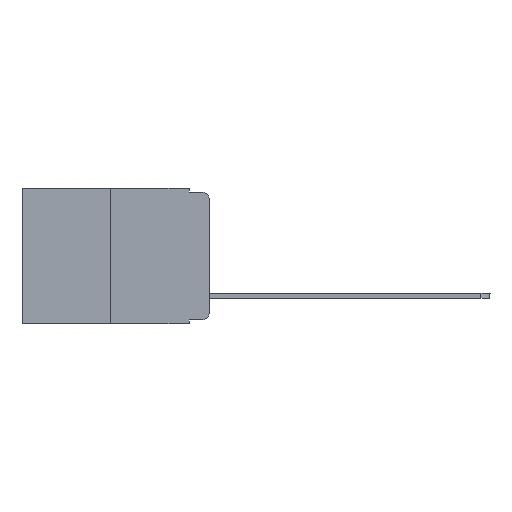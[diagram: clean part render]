
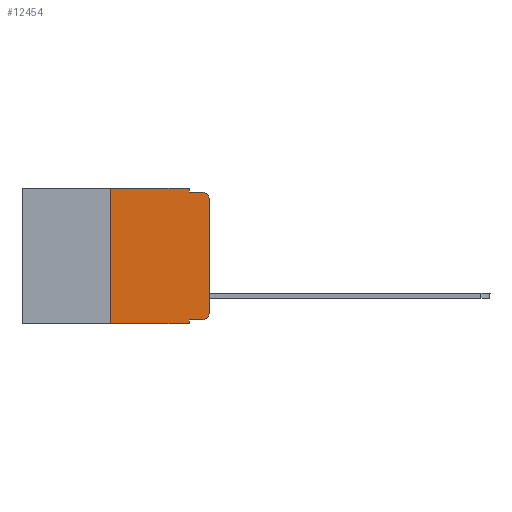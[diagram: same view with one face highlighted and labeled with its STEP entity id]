
A CAD part, left-side view. The second image highlights one B-rep face of the part: STEP entity #12454.
In plain terms, the highlighted planar face has unit normal (-1, 0, 0).
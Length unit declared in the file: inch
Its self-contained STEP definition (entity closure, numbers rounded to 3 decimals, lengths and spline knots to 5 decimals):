
#267 = DIRECTION ( 'NONE',  ( 0., 0., -1. ) ) ;
#279 = FACE_OUTER_BOUND ( 'NONE', #4727, .T. ) ;
#537 = CARTESIAN_POINT ( 'NONE',  ( 0., 0.25, -0.343 ) ) ;
#823 = CARTESIAN_POINT ( 'NONE',  ( 0., 0.051, -0.01 ) ) ;
#937 = DIRECTION ( 'NONE',  ( 0., 0., -1. ) ) ;
#1049 = VECTOR ( 'NONE', #5866, 39.37008 ) ;
#1143 = LINE ( 'NONE', #20910, #19059 ) ;
#1323 = CARTESIAN_POINT ( 'NONE',  ( 0., 0.02, -0.333 ) ) ;
#1586 = ORIENTED_EDGE ( 'NONE', *, *, #7653, .T. ) ;
#2081 = VECTOR ( 'NONE', #16300, 39.37008 ) ;
#2271 = VERTEX_POINT ( 'NONE', #14777 ) ;
#2594 = EDGE_CURVE ( 'NONE', #22328, #10674, #8433, .T. ) ;
#2928 = PLANE ( 'NONE',  #20676 ) ;
#3011 = ORIENTED_EDGE ( 'NONE', *, *, #5702, .F. ) ;
#3160 = CARTESIAN_POINT ( 'NONE',  ( 0., 0., -0.313 ) ) ;
#3504 = EDGE_CURVE ( 'NONE', #10674, #11081, #6456, .T. ) ;
#3681 = DIRECTION ( 'NONE',  ( 0., 0., 1. ) ) ;
#3703 = ORIENTED_EDGE ( 'NONE', *, *, #4003, .F. ) ;
#3707 = EDGE_CURVE ( 'NONE', #8297, #18809, #19769, .T. ) ;
#3853 = DIRECTION ( 'NONE',  ( -1., 0., 0. ) ) ;
#4003 = EDGE_CURVE ( 'NONE', #18809, #17124, #11344, .T. ) ;
#4216 = CARTESIAN_POINT ( 'NONE',  ( 0., 0.051, 0. ) ) ;
#4232 = DIRECTION ( 'NONE',  ( 0., 0., -1. ) ) ;
#4534 = DIRECTION ( 'NONE',  ( -1., 0., 0. ) ) ;
#4727 = EDGE_LOOP ( 'NONE', ( #17742, #10863, #9077, #3703, #17565, #3011, #20948, #12377, #1586, #6518 ) ) ;
#4800 = EDGE_CURVE ( 'NONE', #17124, #2271, #5360, .T. ) ;
#5360 = LINE ( 'NONE', #823, #9434 ) ;
#5702 = EDGE_CURVE ( 'NONE', #21462, #8297, #20244, .T. ) ;
#5766 = EDGE_CURVE ( 'NONE', #17418, #16023, #17217, .T. ) ;
#5866 = DIRECTION ( 'NONE',  ( 0., -1., 0. ) ) ;
#5897 = CARTESIAN_POINT ( 'NONE',  ( 0., 0.25, 0. ) ) ;
#6114 = CARTESIAN_POINT ( 'NONE',  ( 0., 0.02, -0.313 ) ) ;
#6185 = VECTOR ( 'NONE', #3681, 39.37008 ) ;
#6456 = LINE ( 'NONE', #17328, #6185 ) ;
#6518 = ORIENTED_EDGE ( 'NONE', *, *, #2594, .T. ) ;
#7080 = EDGE_CURVE ( 'NONE', #11081, #2271, #10148, .T. ) ;
#7615 = AXIS2_PLACEMENT_3D ( 'NONE', #17784, #3853, #267 ) ;
#7647 = CARTESIAN_POINT ( 'NONE',  ( 0., 0.051, -0.01 ) ) ;
#7653 = EDGE_CURVE ( 'NONE', #17418, #22328, #1143, .T. ) ;
#7744 = DIRECTION ( 'NONE',  ( 0., -1., 0. ) ) ;
#8297 = VERTEX_POINT ( 'NONE', #21191 ) ;
#8433 = CIRCLE ( 'NONE', #11158, 0.02 ) ;
#9013 = CARTESIAN_POINT ( 'NONE',  ( 0., 0.051, -0.343 ) ) ;
#9015 = CARTESIAN_POINT ( 'NONE',  ( 0., 0.051, -0.333 ) ) ;
#9077 = ORIENTED_EDGE ( 'NONE', *, *, #4800, .F. ) ;
#9255 = DIRECTION ( 'NONE',  ( 0., 0., 1. ) ) ;
#9434 = VECTOR ( 'NONE', #7744, 39.37008 ) ;
#9461 = EDGE_CURVE ( 'NONE', #21462, #16023, #21639, .T. ) ;
#9696 = CARTESIAN_POINT ( 'NONE',  ( 0., 0.473, 0. ) ) ;
#10148 = CIRCLE ( 'NONE', #7615, 0.02 ) ;
#10589 = DIRECTION ( 'NONE',  ( 0., -1., 0. ) ) ;
#10674 = VERTEX_POINT ( 'NONE', #3160 ) ;
#10863 = ORIENTED_EDGE ( 'NONE', *, *, #7080, .T. ) ;
#11081 = VERTEX_POINT ( 'NONE', #14730 ) ;
#11119 = CARTESIAN_POINT ( 'NONE',  ( 0., 0.051, 0. ) ) ;
#11125 = CARTESIAN_POINT ( 'NONE',  ( 0., 0.051, 0. ) ) ;
#11158 = AXIS2_PLACEMENT_3D ( 'NONE', #6114, #4534, #16641 ) ;
#11344 = LINE ( 'NONE', #4216, #17839 ) ;
#12365 = VECTOR ( 'NONE', #4232, 39.37008 ) ;
#12377 = ORIENTED_EDGE ( 'NONE', *, *, #5766, .F. ) ;
#12454 = ADVANCED_FACE ( 'NONE', ( #279 ), #2928, .F. ) ;
#12939 = DIRECTION ( 'NONE',  ( 0., 0., -1. ) ) ;
#14519 = VECTOR ( 'NONE', #9255, 39.37008 ) ;
#14730 = CARTESIAN_POINT ( 'NONE',  ( 0., 0., -0.03 ) ) ;
#14777 = CARTESIAN_POINT ( 'NONE',  ( 0., 0.02, -0.01 ) ) ;
#15057 = DIRECTION ( 'NONE',  ( 1., 0., 0. ) ) ;
#16023 = VERTEX_POINT ( 'NONE', #9013 ) ;
#16244 = CARTESIAN_POINT ( 'NONE',  ( 0., 0.473, 0. ) ) ;
#16300 = DIRECTION ( 'NONE',  ( 0., -1., 0. ) ) ;
#16641 = DIRECTION ( 'NONE',  ( 0., 0., -1. ) ) ;
#17124 = VERTEX_POINT ( 'NONE', #7647 ) ;
#17217 = LINE ( 'NONE', #11119, #12365 ) ;
#17328 = CARTESIAN_POINT ( 'NONE',  ( 0., 0., 0. ) ) ;
#17418 = VERTEX_POINT ( 'NONE', #9015 ) ;
#17565 = ORIENTED_EDGE ( 'NONE', *, *, #3707, .F. ) ;
#17742 = ORIENTED_EDGE ( 'NONE', *, *, #3504, .T. ) ;
#17784 = CARTESIAN_POINT ( 'NONE',  ( 0., 0.02, -0.03 ) ) ;
#17839 = VECTOR ( 'NONE', #12939, 39.37008 ) ;
#17892 = CARTESIAN_POINT ( 'NONE',  ( 0., 0.473, -0.343 ) ) ;
#18809 = VERTEX_POINT ( 'NONE', #11125 ) ;
#19059 = VECTOR ( 'NONE', #10589, 39.37008 ) ;
#19769 = LINE ( 'NONE', #16244, #1049 ) ;
#20244 = LINE ( 'NONE', #5897, #14519 ) ;
#20676 = AXIS2_PLACEMENT_3D ( 'NONE', #9696, #15057, #937 ) ;
#20910 = CARTESIAN_POINT ( 'NONE',  ( 0., 0.051, -0.333 ) ) ;
#20948 = ORIENTED_EDGE ( 'NONE', *, *, #9461, .T. ) ;
#21191 = CARTESIAN_POINT ( 'NONE',  ( 0., 0.25, 0. ) ) ;
#21462 = VERTEX_POINT ( 'NONE', #537 ) ;
#21639 = LINE ( 'NONE', #17892, #2081 ) ;
#22328 = VERTEX_POINT ( 'NONE', #1323 ) ;
